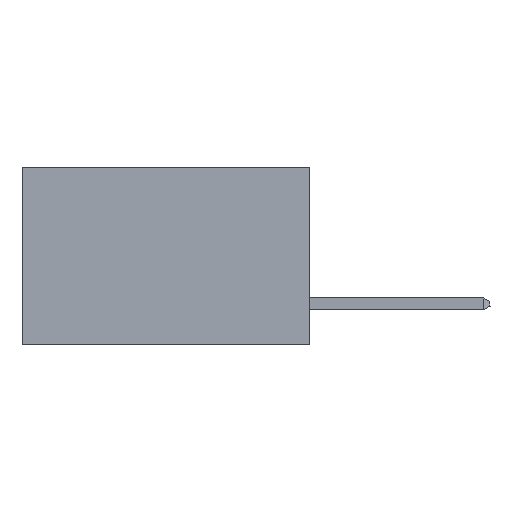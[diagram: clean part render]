
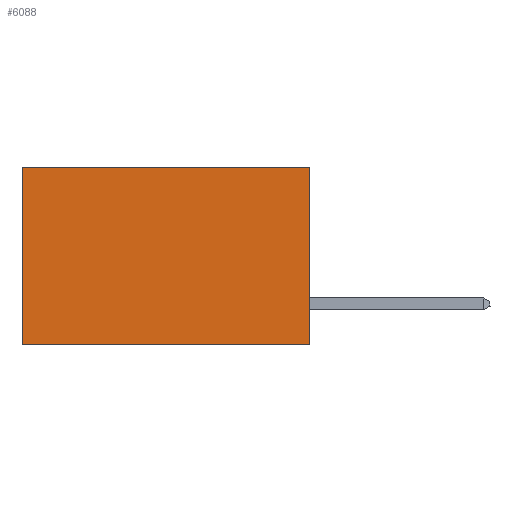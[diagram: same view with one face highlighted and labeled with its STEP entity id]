
A CAD part, left-side view. The second image highlights one B-rep face of the part: STEP entity #6088.
In plain terms, the highlighted planar face has unit normal (-1, 0, 0).
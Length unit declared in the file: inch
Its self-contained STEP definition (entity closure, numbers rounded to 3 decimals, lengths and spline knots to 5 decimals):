
#165 = ORIENTED_EDGE ( 'NONE', *, *, #1403, .F. ) ;
#257 = EDGE_CURVE ( 'NONE', #6013, #3349, #3224, .T. ) ;
#464 = LINE ( 'NONE', #1145, #4650 ) ;
#743 = VERTEX_POINT ( 'NONE', #5927 ) ;
#805 = ORIENTED_EDGE ( 'NONE', *, *, #257, .T. ) ;
#903 = EDGE_CURVE ( 'NONE', #7871, #743, #464, .T. ) ;
#1098 = CARTESIAN_POINT ( 'NONE',  ( 0.2875, 0., 0. ) ) ;
#1112 = DIRECTION ( 'NONE',  ( 0., 1., 0. ) ) ;
#1145 = CARTESIAN_POINT ( 'NONE',  ( 0.2875, 0., -0.37 ) ) ;
#1403 = EDGE_CURVE ( 'NONE', #6013, #7871, #3201, .T. ) ;
#1540 = ORIENTED_EDGE ( 'NONE', *, *, #903, .F. ) ;
#1792 = VECTOR ( 'NONE', #2711, 39.37008 ) ;
#2711 = DIRECTION ( 'NONE',  ( 0., 1., 0. ) ) ;
#3094 = VECTOR ( 'NONE', #3260, 39.37008 ) ;
#3201 = LINE ( 'NONE', #8112, #3094 ) ;
#3224 = LINE ( 'NONE', #7042, #1792 ) ;
#3260 = DIRECTION ( 'NONE',  ( 0., 0., -1. ) ) ;
#3349 = VERTEX_POINT ( 'NONE', #8949 ) ;
#3555 = FACE_OUTER_BOUND ( 'NONE', #6836, .T. ) ;
#3742 = EDGE_CURVE ( 'NONE', #3349, #743, #7803, .T. ) ;
#3989 = CARTESIAN_POINT ( 'NONE',  ( 0.2875, 0.6, 0. ) ) ;
#4292 = DIRECTION ( 'NONE',  ( 0., 0., -1. ) ) ;
#4638 = ORIENTED_EDGE ( 'NONE', *, *, #3742, .T. ) ;
#4650 = VECTOR ( 'NONE', #1112, 39.37008 ) ;
#5927 = CARTESIAN_POINT ( 'NONE',  ( 0.2875, 0.6, -0.37 ) ) ;
#6013 = VERTEX_POINT ( 'NONE', #1098 ) ;
#6088 = ADVANCED_FACE ( 'NONE', ( #3555 ), #8171, .F. ) ;
#6455 = AXIS2_PLACEMENT_3D ( 'NONE', #7514, #8137, #8200 ) ;
#6836 = EDGE_LOOP ( 'NONE', ( #4638, #1540, #165, #805 ) ) ;
#7042 = CARTESIAN_POINT ( 'NONE',  ( 0.2875, 0., 0. ) ) ;
#7182 = CARTESIAN_POINT ( 'NONE',  ( 0.2875, 0., -0.37 ) ) ;
#7514 = CARTESIAN_POINT ( 'NONE',  ( 0.2875, 0., 0. ) ) ;
#7803 = LINE ( 'NONE', #3989, #8450 ) ;
#7871 = VERTEX_POINT ( 'NONE', #7182 ) ;
#8112 = CARTESIAN_POINT ( 'NONE',  ( 0.2875, 0., 0. ) ) ;
#8137 = DIRECTION ( 'NONE',  ( 1., 0., 0. ) ) ;
#8171 = PLANE ( 'NONE',  #6455 ) ;
#8200 = DIRECTION ( 'NONE',  ( 0., 0., -1. ) ) ;
#8450 = VECTOR ( 'NONE', #4292, 39.37008 ) ;
#8949 = CARTESIAN_POINT ( 'NONE',  ( 0.2875, 0.6, 0. ) ) ;
